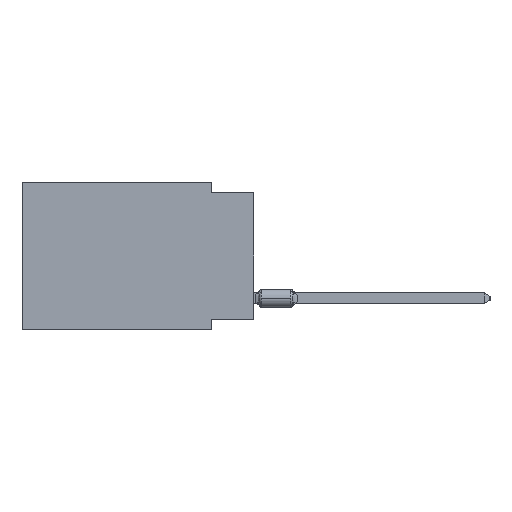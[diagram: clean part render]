
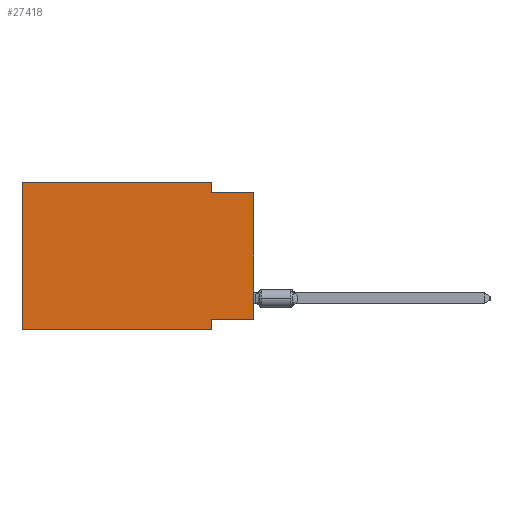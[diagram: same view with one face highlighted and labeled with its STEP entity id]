
A CAD part, left-side view. The second image highlights one B-rep face of the part: STEP entity #27418.
In plain terms, the highlighted planar face has unit normal (-1, 0, 0).
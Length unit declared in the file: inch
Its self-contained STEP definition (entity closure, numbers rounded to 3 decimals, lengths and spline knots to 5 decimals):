
#1229 = ORIENTED_EDGE ( 'NONE', *, *, #81310, .F. ) ;
#3495 = ORIENTED_EDGE ( 'NONE', *, *, #67794, .F. ) ;
#4310 = VERTEX_POINT ( 'NONE', #18146 ) ;
#4504 = ORIENTED_EDGE ( 'NONE', *, *, #67566, .T. ) ;
#5475 = CARTESIAN_POINT ( 'NONE',  ( 0., 0.55, -0.35 ) ) ;
#7478 = LINE ( 'NONE', #108055, #28464 ) ;
#8512 = AXIS2_PLACEMENT_3D ( 'NONE', #78773, #46842, #29276 ) ;
#10220 = VERTEX_POINT ( 'NONE', #12913 ) ;
#10904 = CARTESIAN_POINT ( 'NONE',  ( 0., 0.55, 0. ) ) ;
#10927 = CARTESIAN_POINT ( 'NONE',  ( 0., 0.1, -0.35 ) ) ;
#12198 = ORIENTED_EDGE ( 'NONE', *, *, #35711, .T. ) ;
#12913 = CARTESIAN_POINT ( 'NONE',  ( 0., 0., -0.025 ) ) ;
#16094 = DIRECTION ( 'NONE',  ( 0., -1., 0. ) ) ;
#18101 = DIRECTION ( 'NONE',  ( 0., 0., -1. ) ) ;
#18146 = CARTESIAN_POINT ( 'NONE',  ( 0., 0.1, 0. ) ) ;
#21321 = CARTESIAN_POINT ( 'NONE',  ( 0., 0.1, -0.025 ) ) ;
#22887 = CARTESIAN_POINT ( 'NONE',  ( 0., 0., 0. ) ) ;
#26991 = VECTOR ( 'NONE', #27827, 39.37008 ) ;
#27025 = VERTEX_POINT ( 'NONE', #29942 ) ;
#27418 = ADVANCED_FACE ( 'NONE', ( #96892 ), #87565, .F. ) ;
#27827 = DIRECTION ( 'NONE',  ( 0., 1., 0. ) ) ;
#28464 = VECTOR ( 'NONE', #66288, 39.37008 ) ;
#29276 = DIRECTION ( 'NONE',  ( 0., 0., -1. ) ) ;
#29863 = VERTEX_POINT ( 'NONE', #5475 ) ;
#29942 = CARTESIAN_POINT ( 'NONE',  ( 0., 0.55, 0. ) ) ;
#33369 = VECTOR ( 'NONE', #98697, 39.37008 ) ;
#35711 = EDGE_CURVE ( 'NONE', #29863, #105696, #51261, .T. ) ;
#36461 = VECTOR ( 'NONE', #102174, 39.37008 ) ;
#37576 = EDGE_LOOP ( 'NONE', ( #4504, #76452, #3495, #96191, #45801, #12198, #1229, #75322 ) ) ;
#40402 = CARTESIAN_POINT ( 'NONE',  ( 0., 0.55, 0. ) ) ;
#41484 = LINE ( 'NONE', #40402, #33369 ) ;
#42378 = DIRECTION ( 'NONE',  ( 0., -1., 0. ) ) ;
#42438 = VERTEX_POINT ( 'NONE', #85708 ) ;
#43467 = LINE ( 'NONE', #76468, #76619 ) ;
#45801 = ORIENTED_EDGE ( 'NONE', *, *, #96274, .F. ) ;
#46842 = DIRECTION ( 'NONE',  ( 1., 0., 0. ) ) ;
#46968 = EDGE_CURVE ( 'NONE', #51968, #10220, #43467, .T. ) ;
#48494 = VECTOR ( 'NONE', #16094, 39.37008 ) ;
#50570 = CARTESIAN_POINT ( 'NONE',  ( 0., 0., -0.325 ) ) ;
#51261 = LINE ( 'NONE', #58419, #48494 ) ;
#51968 = VERTEX_POINT ( 'NONE', #21321 ) ;
#52567 = CARTESIAN_POINT ( 'NONE',  ( 0., 0., -0.325 ) ) ;
#58419 = CARTESIAN_POINT ( 'NONE',  ( 0., 0.55, -0.35 ) ) ;
#61491 = LINE ( 'NONE', #10927, #78173 ) ;
#61830 = VECTOR ( 'NONE', #97116, 39.37008 ) ;
#66288 = DIRECTION ( 'NONE',  ( 0., 0., -1. ) ) ;
#67566 = EDGE_CURVE ( 'NONE', #79284, #10220, #96569, .T. ) ;
#67794 = EDGE_CURVE ( 'NONE', #4310, #51968, #7478, .T. ) ;
#69721 = LINE ( 'NONE', #10904, #36461 ) ;
#71054 = EDGE_CURVE ( 'NONE', #79284, #42438, #94358, .T. ) ;
#73646 = EDGE_CURVE ( 'NONE', #27025, #4310, #41484, .T. ) ;
#75322 = ORIENTED_EDGE ( 'NONE', *, *, #71054, .F. ) ;
#76452 = ORIENTED_EDGE ( 'NONE', *, *, #46968, .F. ) ;
#76468 = CARTESIAN_POINT ( 'NONE',  ( 0., 0., -0.025 ) ) ;
#76619 = VECTOR ( 'NONE', #42378, 39.37008 ) ;
#78173 = VECTOR ( 'NONE', #18101, 39.37008 ) ;
#78773 = CARTESIAN_POINT ( 'NONE',  ( 0., 0.55, 0. ) ) ;
#79284 = VERTEX_POINT ( 'NONE', #50570 ) ;
#80081 = CARTESIAN_POINT ( 'NONE',  ( 0., 0.1, -0.35 ) ) ;
#81310 = EDGE_CURVE ( 'NONE', #42438, #105696, #61491, .T. ) ;
#85708 = CARTESIAN_POINT ( 'NONE',  ( 0., 0.1, -0.325 ) ) ;
#87565 = PLANE ( 'NONE',  #8512 ) ;
#94358 = LINE ( 'NONE', #52567, #26991 ) ;
#96191 = ORIENTED_EDGE ( 'NONE', *, *, #73646, .F. ) ;
#96274 = EDGE_CURVE ( 'NONE', #29863, #27025, #69721, .T. ) ;
#96569 = LINE ( 'NONE', #22887, #61830 ) ;
#96892 = FACE_OUTER_BOUND ( 'NONE', #37576, .T. ) ;
#97116 = DIRECTION ( 'NONE',  ( 0., 0., 1. ) ) ;
#98697 = DIRECTION ( 'NONE',  ( 0., -1., 0. ) ) ;
#102174 = DIRECTION ( 'NONE',  ( 0., 0., 1. ) ) ;
#105696 = VERTEX_POINT ( 'NONE', #80081 ) ;
#108055 = CARTESIAN_POINT ( 'NONE',  ( 0., 0.1, 0. ) ) ;
